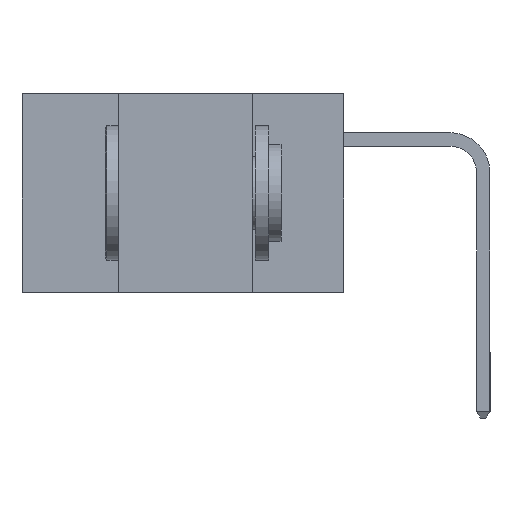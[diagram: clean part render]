
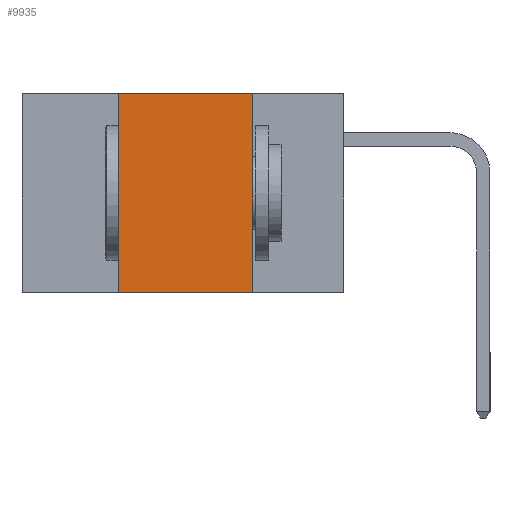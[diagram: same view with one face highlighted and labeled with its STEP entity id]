
A CAD part, left-side view. The second image highlights one B-rep face of the part: STEP entity #9935.
In plain terms, the highlighted planar face has unit normal (-1, 0, 0).
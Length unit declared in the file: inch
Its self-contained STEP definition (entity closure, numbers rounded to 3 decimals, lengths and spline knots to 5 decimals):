
#124 = CARTESIAN_POINT ( 'NONE',  ( 0., 0.6, -0.37 ) ) ;
#976 = DIRECTION ( 'NONE',  ( 0., -1., 0. ) ) ;
#1446 = EDGE_CURVE ( 'NONE', #11709, #9289, #7701, .T. ) ;
#2053 = FACE_OUTER_BOUND ( 'NONE', #13286, .T. ) ;
#2124 = ORIENTED_EDGE ( 'NONE', *, *, #8548, .F. ) ;
#2166 = VERTEX_POINT ( 'NONE', #6194 ) ;
#2230 = CARTESIAN_POINT ( 'NONE',  ( 0., 0.17, 0. ) ) ;
#2606 = ORIENTED_EDGE ( 'NONE', *, *, #12659, .T. ) ;
#2704 = DIRECTION ( 'NONE',  ( 0., 0., -1. ) ) ;
#3043 = LINE ( 'NONE', #12007, #12128 ) ;
#4225 = DIRECTION ( 'NONE',  ( 0., 0., -1. ) ) ;
#4978 = ORIENTED_EDGE ( 'NONE', *, *, #12745, .F. ) ;
#5285 = PLANE ( 'NONE',  #6715 ) ;
#5958 = VERTEX_POINT ( 'NONE', #2230 ) ;
#6194 = CARTESIAN_POINT ( 'NONE',  ( 0., 0.17, -0.37 ) ) ;
#6705 = DIRECTION ( 'NONE',  ( 0., 0., 1. ) ) ;
#6715 = AXIS2_PLACEMENT_3D ( 'NONE', #9617, #13955, #4225 ) ;
#6917 = ORIENTED_EDGE ( 'NONE', *, *, #1446, .F. ) ;
#7701 = LINE ( 'NONE', #9885, #11822 ) ;
#8548 = EDGE_CURVE ( 'NONE', #9289, #5958, #3043, .T. ) ;
#8772 = DIRECTION ( 'NONE',  ( 0., -1., 0. ) ) ;
#9289 = VERTEX_POINT ( 'NONE', #11632 ) ;
#9617 = CARTESIAN_POINT ( 'NONE',  ( 0., 0.6, 0. ) ) ;
#9835 = LINE ( 'NONE', #124, #12880 ) ;
#9885 = CARTESIAN_POINT ( 'NONE',  ( 0., 0.42, -0.37 ) ) ;
#9935 = ADVANCED_FACE ( 'NONE', ( #2053 ), #5285, .F. ) ;
#10166 = VECTOR ( 'NONE', #2704, 39.37008 ) ;
#10197 = CARTESIAN_POINT ( 'NONE',  ( 0., 0.17, -0.37 ) ) ;
#10599 = CARTESIAN_POINT ( 'NONE',  ( 0., 0.42, -0.37 ) ) ;
#11135 = LINE ( 'NONE', #10197, #10166 ) ;
#11632 = CARTESIAN_POINT ( 'NONE',  ( 0., 0.42, 0. ) ) ;
#11709 = VERTEX_POINT ( 'NONE', #10599 ) ;
#11822 = VECTOR ( 'NONE', #6705, 39.37008 ) ;
#12007 = CARTESIAN_POINT ( 'NONE',  ( 0., 0.6, 0. ) ) ;
#12128 = VECTOR ( 'NONE', #976, 39.37008 ) ;
#12659 = EDGE_CURVE ( 'NONE', #11709, #2166, #9835, .T. ) ;
#12745 = EDGE_CURVE ( 'NONE', #5958, #2166, #11135, .T. ) ;
#12880 = VECTOR ( 'NONE', #8772, 39.37008 ) ;
#13286 = EDGE_LOOP ( 'NONE', ( #4978, #2124, #6917, #2606 ) ) ;
#13955 = DIRECTION ( 'NONE',  ( 1., 0., 0. ) ) ;
